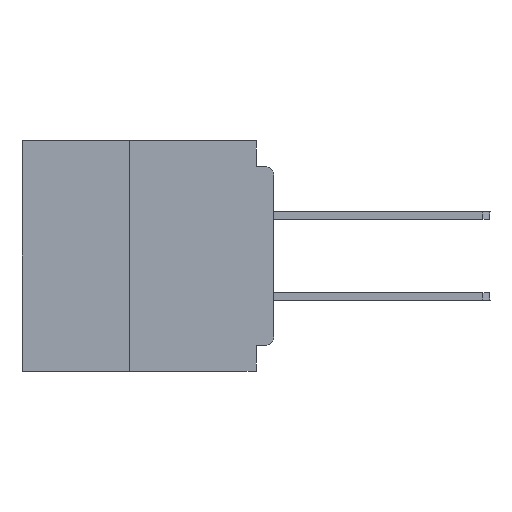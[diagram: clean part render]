
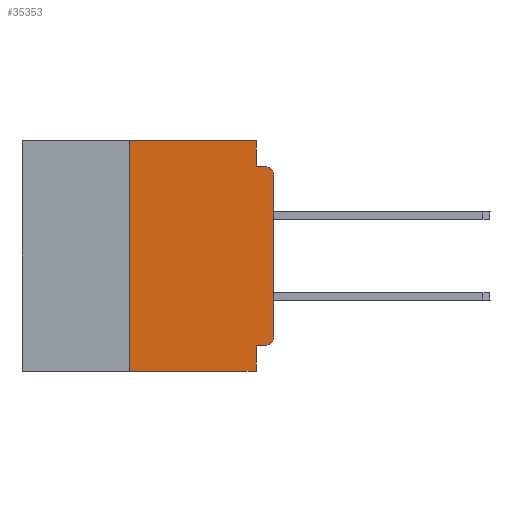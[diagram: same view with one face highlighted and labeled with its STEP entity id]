
A CAD part, left-side view. The second image highlights one B-rep face of the part: STEP entity #35353.
In plain terms, the highlighted planar face has unit normal (-1, 0, 0).
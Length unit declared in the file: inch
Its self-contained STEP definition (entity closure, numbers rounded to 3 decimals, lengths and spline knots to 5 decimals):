
#1084 = DIRECTION ( 'NONE',  ( 0., 0., -1. ) ) ;
#1875 = CARTESIAN_POINT ( 'NONE',  ( 0., 0., 0. ) ) ;
#2381 = CARTESIAN_POINT ( 'NONE',  ( 0., 0.015, -0.06 ) ) ;
#2431 = ORIENTED_EDGE ( 'NONE', *, *, #56138, .F. ) ;
#2547 = ORIENTED_EDGE ( 'NONE', *, *, #16808, .F. ) ;
#2991 = DIRECTION ( 'NONE',  ( 0., 0., -1. ) ) ;
#3040 = EDGE_CURVE ( 'NONE', #46433, #30199, #47791, .T. ) ;
#4679 = CARTESIAN_POINT ( 'NONE',  ( 0., 0.015, -0.045 ) ) ;
#5586 = CARTESIAN_POINT ( 'NONE',  ( 0., 0.437, 0. ) ) ;
#5694 = LINE ( 'NONE', #26790, #7140 ) ;
#5856 = CARTESIAN_POINT ( 'NONE',  ( 0., 0.015, -0.355 ) ) ;
#6286 = DIRECTION ( 'NONE',  ( 0., 0., -1. ) ) ;
#6744 = EDGE_CURVE ( 'NONE', #31500, #59654, #35633, .T. ) ;
#6839 = LINE ( 'NONE', #10387, #41289 ) ;
#7040 = DIRECTION ( 'NONE',  ( 0., 0., -1. ) ) ;
#7140 = VECTOR ( 'NONE', #40927, 39.37008 ) ;
#8536 = CARTESIAN_POINT ( 'NONE',  ( 0., 0.25, -0.4 ) ) ;
#8629 = VERTEX_POINT ( 'NONE', #22390 ) ;
#9829 = VECTOR ( 'NONE', #34614, 39.37008 ) ;
#10279 = PLANE ( 'NONE',  #19231 ) ;
#10387 = CARTESIAN_POINT ( 'NONE',  ( 0., 0.437, -0.4 ) ) ;
#10461 = VECTOR ( 'NONE', #20264, 39.37008 ) ;
#10868 = EDGE_CURVE ( 'NONE', #59654, #53429, #58151, .T. ) ;
#11302 = ORIENTED_EDGE ( 'NONE', *, *, #33043, .T. ) ;
#11402 = EDGE_CURVE ( 'NONE', #32603, #46604, #6839, .T. ) ;
#13499 = EDGE_CURVE ( 'NONE', #30199, #8629, #32955, .T. ) ;
#15080 = DIRECTION ( 'NONE',  ( 0., -1., 0. ) ) ;
#16808 = EDGE_CURVE ( 'NONE', #8629, #20691, #42968, .T. ) ;
#17654 = CARTESIAN_POINT ( 'NONE',  ( 0., 0.031, -0.4 ) ) ;
#17703 = EDGE_CURVE ( 'NONE', #58569, #46604, #27469, .T. ) ;
#19231 = AXIS2_PLACEMENT_3D ( 'NONE', #5586, #29118, #1084 ) ;
#19865 = AXIS2_PLACEMENT_3D ( 'NONE', #59008, #31019, #2991 ) ;
#20207 = DIRECTION ( 'NONE',  ( 0., -1., 0. ) ) ;
#20259 = ORIENTED_EDGE ( 'NONE', *, *, #13499, .F. ) ;
#20264 = DIRECTION ( 'NONE',  ( 0., -1., 0. ) ) ;
#20472 = VECTOR ( 'NONE', #6286, 39.37008 ) ;
#20691 = VERTEX_POINT ( 'NONE', #4679 ) ;
#21003 = CARTESIAN_POINT ( 'NONE',  ( 0., 0.437, 0. ) ) ;
#21313 = CARTESIAN_POINT ( 'NONE',  ( 0., 0.031, -0.4 ) ) ;
#21590 = CARTESIAN_POINT ( 'NONE',  ( 0., 0., -0.34 ) ) ;
#22390 = CARTESIAN_POINT ( 'NONE',  ( 0., 0.031, -0.045 ) ) ;
#23884 = ORIENTED_EDGE ( 'NONE', *, *, #17703, .F. ) ;
#24620 = CARTESIAN_POINT ( 'NONE',  ( 0., 0.25, 0. ) ) ;
#26456 = AXIS2_PLACEMENT_3D ( 'NONE', #2381, #35114, #7040 ) ;
#26525 = CARTESIAN_POINT ( 'NONE',  ( 0., 0.031, -0.355 ) ) ;
#26790 = CARTESIAN_POINT ( 'NONE',  ( 0., 0., -0.355 ) ) ;
#27432 = ORIENTED_EDGE ( 'NONE', *, *, #35489, .F. ) ;
#27469 = LINE ( 'NONE', #17654, #28923 ) ;
#28923 = VECTOR ( 'NONE', #50407, 39.37008 ) ;
#29118 = DIRECTION ( 'NONE',  ( 1., 0., 0. ) ) ;
#29343 = CARTESIAN_POINT ( 'NONE',  ( 0., 0.031, 0. ) ) ;
#30199 = VERTEX_POINT ( 'NONE', #29343 ) ;
#31019 = DIRECTION ( 'NONE',  ( -1., 0., 0. ) ) ;
#31500 = VERTEX_POINT ( 'NONE', #5856 ) ;
#32603 = VERTEX_POINT ( 'NONE', #36611 ) ;
#32955 = LINE ( 'NONE', #39061, #20472 ) ;
#33023 = CARTESIAN_POINT ( 'NONE',  ( 0., 0., -0.06 ) ) ;
#33043 = EDGE_CURVE ( 'NONE', #53429, #20691, #36998, .T. ) ;
#34348 = CARTESIAN_POINT ( 'NONE',  ( 0., 0., -0.045 ) ) ;
#34537 = EDGE_LOOP ( 'NONE', ( #37497, #11302, #2547, #20259, #38478, #27432, #37738, #23884, #2431, #55673 ) ) ;
#34580 = FACE_OUTER_BOUND ( 'NONE', #34537, .T. ) ;
#34614 = DIRECTION ( 'NONE',  ( 0., 0., 1. ) ) ;
#35114 = DIRECTION ( 'NONE',  ( -1., 0., 0. ) ) ;
#35353 = ADVANCED_FACE ( 'NONE', ( #34580 ), #10279, .F. ) ;
#35489 = EDGE_CURVE ( 'NONE', #32603, #46433, #60154, .T. ) ;
#35633 = CIRCLE ( 'NONE', #19865, 0.015 ) ;
#36611 = CARTESIAN_POINT ( 'NONE',  ( 0., 0.25, -0.4 ) ) ;
#36998 = CIRCLE ( 'NONE', #26456, 0.015 ) ;
#37497 = ORIENTED_EDGE ( 'NONE', *, *, #10868, .T. ) ;
#37738 = ORIENTED_EDGE ( 'NONE', *, *, #11402, .T. ) ;
#38478 = ORIENTED_EDGE ( 'NONE', *, *, #3040, .F. ) ;
#39061 = CARTESIAN_POINT ( 'NONE',  ( 0., 0.031, 0. ) ) ;
#40927 = DIRECTION ( 'NONE',  ( 0., 1., 0. ) ) ;
#41289 = VECTOR ( 'NONE', #15080, 39.37008 ) ;
#41297 = DIRECTION ( 'NONE',  ( 0., 0., 1. ) ) ;
#42968 = LINE ( 'NONE', #34348, #56855 ) ;
#46433 = VERTEX_POINT ( 'NONE', #24620 ) ;
#46604 = VERTEX_POINT ( 'NONE', #21313 ) ;
#47694 = VECTOR ( 'NONE', #41297, 39.37008 ) ;
#47791 = LINE ( 'NONE', #21003, #10461 ) ;
#50407 = DIRECTION ( 'NONE',  ( 0., 0., -1. ) ) ;
#53429 = VERTEX_POINT ( 'NONE', #33023 ) ;
#55673 = ORIENTED_EDGE ( 'NONE', *, *, #6744, .T. ) ;
#56138 = EDGE_CURVE ( 'NONE', #31500, #58569, #5694, .T. ) ;
#56855 = VECTOR ( 'NONE', #20207, 39.37008 ) ;
#58151 = LINE ( 'NONE', #1875, #9829 ) ;
#58569 = VERTEX_POINT ( 'NONE', #26525 ) ;
#59008 = CARTESIAN_POINT ( 'NONE',  ( 0., 0.015, -0.34 ) ) ;
#59654 = VERTEX_POINT ( 'NONE', #21590 ) ;
#60154 = LINE ( 'NONE', #8536, #47694 ) ;
